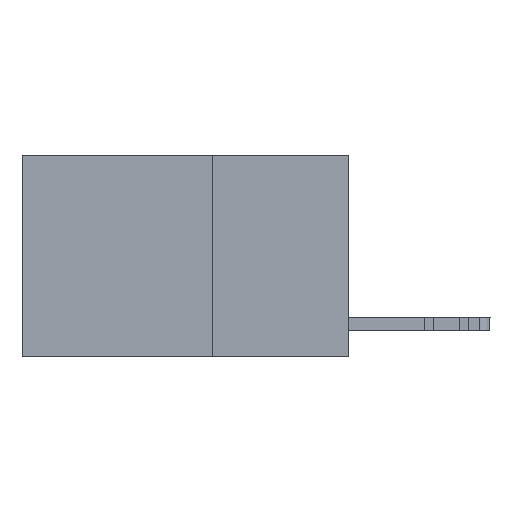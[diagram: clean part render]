
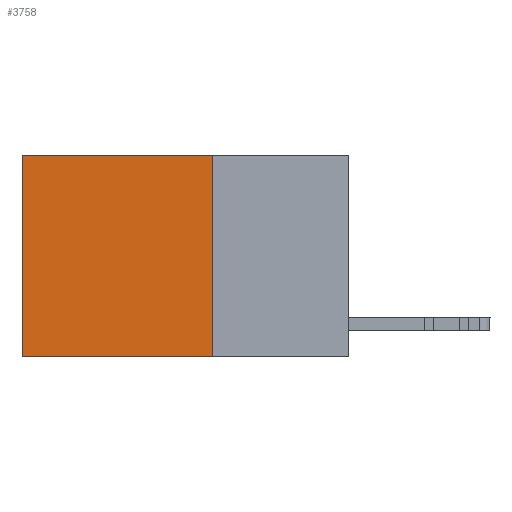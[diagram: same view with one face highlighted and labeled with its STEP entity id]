
A CAD part, left-side view. The second image highlights one B-rep face of the part: STEP entity #3758.
In plain terms, the highlighted planar face has unit normal (-1, 0, 0).
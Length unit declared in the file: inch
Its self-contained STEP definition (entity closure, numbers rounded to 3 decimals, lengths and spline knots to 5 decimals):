
#2041 = CARTESIAN_POINT ( 'NONE',  ( 0.2625, 0.6, -0.37 ) ) ;
#2923 = CARTESIAN_POINT ( 'NONE',  ( 0.2625, 0.25, 0. ) ) ;
#3758 = ADVANCED_FACE ( 'NONE', ( #12703 ), #16310, .F. ) ;
#3935 = EDGE_CURVE ( 'NONE', #26208, #25454, #19711, .T. ) ;
#5207 = DIRECTION ( 'NONE',  ( 1., 0., 0. ) ) ;
#5848 = VECTOR ( 'NONE', #20342, 39.37008 ) ;
#6138 = DIRECTION ( 'NONE',  ( 0., 1., 0. ) ) ;
#6573 = ORIENTED_EDGE ( 'NONE', *, *, #17585, .F. ) ;
#7612 = VECTOR ( 'NONE', #6138, 39.37008 ) ;
#7739 = CARTESIAN_POINT ( 'NONE',  ( 0.2625, 0.6, 0. ) ) ;
#7786 = VECTOR ( 'NONE', #19168, 39.37008 ) ;
#9456 = AXIS2_PLACEMENT_3D ( 'NONE', #2923, #5207, #20825 ) ;
#9672 = CARTESIAN_POINT ( 'NONE',  ( 0.2625, 0.25, -0.37 ) ) ;
#11735 = LINE ( 'NONE', #13562, #5848 ) ;
#12703 = FACE_OUTER_BOUND ( 'NONE', #23583, .T. ) ;
#13401 = ORIENTED_EDGE ( 'NONE', *, *, #28149, .T. ) ;
#13500 = VERTEX_POINT ( 'NONE', #9672 ) ;
#13562 = CARTESIAN_POINT ( 'NONE',  ( 0.2625, 0.25, 0. ) ) ;
#15311 = VECTOR ( 'NONE', #15986, 39.37008 ) ;
#15986 = DIRECTION ( 'NONE',  ( 0., 0., -1. ) ) ;
#16310 = PLANE ( 'NONE',  #9456 ) ;
#16340 = ORIENTED_EDGE ( 'NONE', *, *, #3935, .T. ) ;
#16898 = CARTESIAN_POINT ( 'NONE',  ( 0.2625, 0.25, 0. ) ) ;
#17267 = CARTESIAN_POINT ( 'NONE',  ( 0.2625, 0.25, -0.37 ) ) ;
#17585 = EDGE_CURVE ( 'NONE', #26208, #13500, #11735, .T. ) ;
#19168 = DIRECTION ( 'NONE',  ( 0., 1., 0. ) ) ;
#19711 = LINE ( 'NONE', #16898, #7786 ) ;
#20342 = DIRECTION ( 'NONE',  ( 0., 0., -1. ) ) ;
#20825 = DIRECTION ( 'NONE',  ( 0., 0., -1. ) ) ;
#21073 = VERTEX_POINT ( 'NONE', #2041 ) ;
#21303 = LINE ( 'NONE', #22648, #15311 ) ;
#22363 = CARTESIAN_POINT ( 'NONE',  ( 0.2625, 0.25, 0. ) ) ;
#22648 = CARTESIAN_POINT ( 'NONE',  ( 0.2625, 0.6, 0. ) ) ;
#23583 = EDGE_LOOP ( 'NONE', ( #13401, #23880, #6573, #16340 ) ) ;
#23880 = ORIENTED_EDGE ( 'NONE', *, *, #28016, .F. ) ;
#25392 = LINE ( 'NONE', #17267, #7612 ) ;
#25454 = VERTEX_POINT ( 'NONE', #7739 ) ;
#26208 = VERTEX_POINT ( 'NONE', #22363 ) ;
#28016 = EDGE_CURVE ( 'NONE', #13500, #21073, #25392, .T. ) ;
#28149 = EDGE_CURVE ( 'NONE', #25454, #21073, #21303, .T. ) ;
